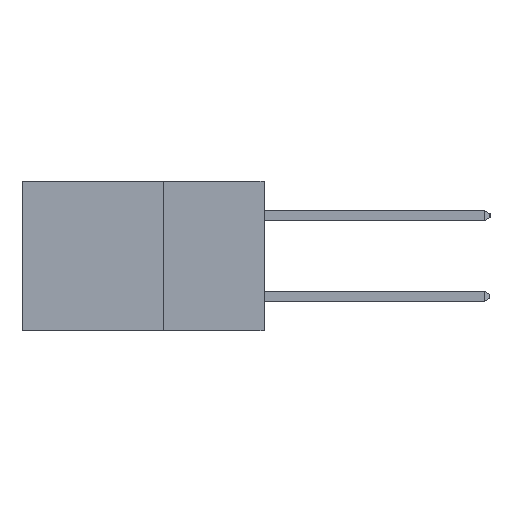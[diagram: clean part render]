
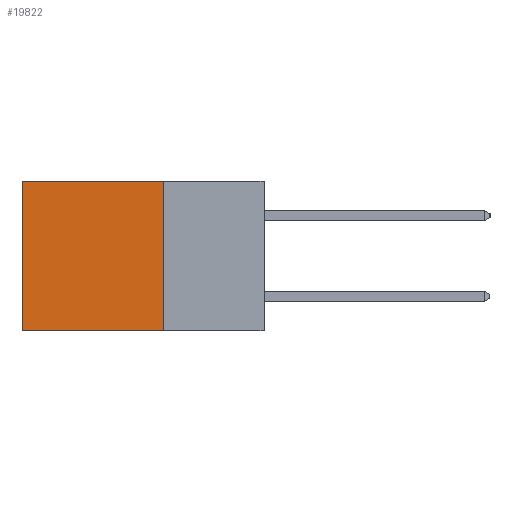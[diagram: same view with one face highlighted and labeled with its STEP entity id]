
A CAD part, left-side view. The second image highlights one B-rep face of the part: STEP entity #19822.
In plain terms, the highlighted planar face has unit normal (-1, 0, 0).
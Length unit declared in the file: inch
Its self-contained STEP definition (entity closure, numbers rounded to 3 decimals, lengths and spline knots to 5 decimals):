
#40 = LINE ( 'NONE', #22356, #8977 ) ;
#256 = LINE ( 'NONE', #7082, #18369 ) ;
#1015 = CARTESIAN_POINT ( 'NONE',  ( 0.2615, 0.6, -0.37 ) ) ;
#1195 = FACE_OUTER_BOUND ( 'NONE', #12771, .T. ) ;
#1365 = CARTESIAN_POINT ( 'NONE',  ( 0.2615, 0.25, 0. ) ) ;
#1613 = VECTOR ( 'NONE', #6920, 39.37008 ) ;
#1618 = DIRECTION ( 'NONE',  ( 0., 1., 0. ) ) ;
#2171 = LINE ( 'NONE', #8606, #6468 ) ;
#2995 = CARTESIAN_POINT ( 'NONE',  ( 0.2615, 0.25, -0.37 ) ) ;
#4859 = DIRECTION ( 'NONE',  ( 0., 0., -1. ) ) ;
#5154 = CARTESIAN_POINT ( 'NONE',  ( 0.2615, 0.25, -0.37 ) ) ;
#6180 = ORIENTED_EDGE ( 'NONE', *, *, #7271, .T. ) ;
#6468 = VECTOR ( 'NONE', #22218, 39.37008 ) ;
#6469 = DIRECTION ( 'NONE',  ( 0., 0., -1. ) ) ;
#6545 = CARTESIAN_POINT ( 'NONE',  ( 0.2615, 0.6, 0. ) ) ;
#6654 = ORIENTED_EDGE ( 'NONE', *, *, #16503, .F. ) ;
#6920 = DIRECTION ( 'NONE',  ( 0., 0., -1. ) ) ;
#7082 = CARTESIAN_POINT ( 'NONE',  ( 0.2615, 0.6, -0.37 ) ) ;
#7271 = EDGE_CURVE ( 'NONE', #10194, #16319, #256, .T. ) ;
#8606 = CARTESIAN_POINT ( 'NONE',  ( 0.2615, 0.25, 0. ) ) ;
#8977 = VECTOR ( 'NONE', #1618, 39.37008 ) ;
#10194 = VERTEX_POINT ( 'NONE', #6545 ) ;
#11166 = EDGE_CURVE ( 'NONE', #18073, #16319, #40, .T. ) ;
#12487 = CARTESIAN_POINT ( 'NONE',  ( 0.2615, 0.25, -0.37 ) ) ;
#12771 = EDGE_LOOP ( 'NONE', ( #6180, #20372, #6654, #20090 ) ) ;
#13578 = PLANE ( 'NONE',  #18709 ) ;
#15298 = DIRECTION ( 'NONE',  ( 1., 0., 0. ) ) ;
#15700 = LINE ( 'NONE', #5154, #1613 ) ;
#16319 = VERTEX_POINT ( 'NONE', #1015 ) ;
#16472 = EDGE_CURVE ( 'NONE', #18557, #10194, #2171, .T. ) ;
#16503 = EDGE_CURVE ( 'NONE', #18557, #18073, #15700, .T. ) ;
#18073 = VERTEX_POINT ( 'NONE', #12487 ) ;
#18369 = VECTOR ( 'NONE', #6469, 39.37008 ) ;
#18557 = VERTEX_POINT ( 'NONE', #1365 ) ;
#18709 = AXIS2_PLACEMENT_3D ( 'NONE', #2995, #15298, #4859 ) ;
#19822 = ADVANCED_FACE ( 'NONE', ( #1195 ), #13578, .F. ) ;
#20090 = ORIENTED_EDGE ( 'NONE', *, *, #16472, .T. ) ;
#20372 = ORIENTED_EDGE ( 'NONE', *, *, #11166, .F. ) ;
#22218 = DIRECTION ( 'NONE',  ( 0., 1., 0. ) ) ;
#22356 = CARTESIAN_POINT ( 'NONE',  ( 0.2615, 0.25, -0.37 ) ) ;
